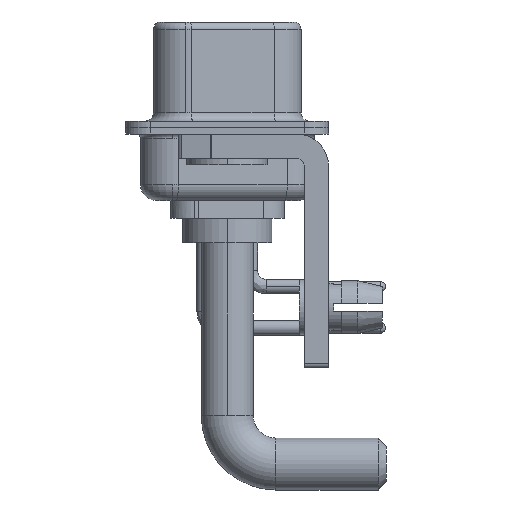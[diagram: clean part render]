
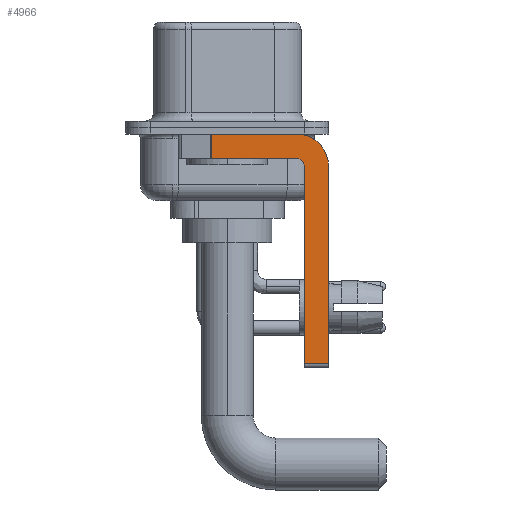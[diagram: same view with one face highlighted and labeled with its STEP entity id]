
A CAD part, left-side view. The second image highlights one B-rep face of the part: STEP entity #4966.
In plain terms, the highlighted planar face has unit normal (-1, 0, 0).
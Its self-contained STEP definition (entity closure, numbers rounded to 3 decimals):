
#356 = EDGE_CURVE ( 'NONE', #11804, #25459, #4008, .T. ) ;
#1149 = CARTESIAN_POINT ( 'NONE',  ( -2.9, 0.978, -1.9 ) ) ;
#2379 = ORIENTED_EDGE ( 'NONE', *, *, #14048, .T. ) ;
#2814 = VECTOR ( 'NONE', #11706, 1000. ) ;
#3312 = DIRECTION ( 'NONE',  ( 0., 0., -1. ) ) ;
#3522 = ORIENTED_EDGE ( 'NONE', *, *, #25595, .F. ) ;
#4008 = LINE ( 'NONE', #19094, #18369 ) ;
#4012 = EDGE_CURVE ( 'NONE', #11804, #10591, #15947, .T. ) ;
#4028 = VECTOR ( 'NONE', #9507, 1000. ) ;
#4048 = DIRECTION ( 'NONE',  ( 0., 0., -1. ) ) ;
#4195 = VERTEX_POINT ( 'NONE', #5942 ) ;
#4743 = ORIENTED_EDGE ( 'NONE', *, *, #9027, .F. ) ;
#4966 = ADVANCED_FACE ( 'NONE', ( #19493 ), #5342, .F. ) ;
#5143 = CARTESIAN_POINT ( 'NONE',  ( -2.9, -4.25, -1.9 ) ) ;
#5342 = PLANE ( 'NONE',  #10728 ) ;
#5614 = CARTESIAN_POINT ( 'NONE',  ( -2.9, -6.25, -2.4 ) ) ;
#5782 = AXIS2_PLACEMENT_3D ( 'NONE', #16795, #25174, #4048 ) ;
#5942 = CARTESIAN_POINT ( 'NONE',  ( -2.9, -4.75, -14.55 ) ) ;
#5973 = DIRECTION ( 'NONE',  ( 0., 1., 0. ) ) ;
#6993 = VECTOR ( 'NONE', #5973, 1000. ) ;
#7260 = CARTESIAN_POINT ( 'NONE',  ( -2.9, -4.25, -2.4 ) ) ;
#7517 = EDGE_LOOP ( 'NONE', ( #22736, #12657, #3522, #9685, #20206, #2379, #23574, #4743 ) ) ;
#8317 = AXIS2_PLACEMENT_3D ( 'NONE', #21967, #15934, #9769 ) ;
#9027 = EDGE_CURVE ( 'NONE', #25459, #19222, #22877, .T. ) ;
#9507 = DIRECTION ( 'NONE',  ( 0., -1., 0. ) ) ;
#9685 = ORIENTED_EDGE ( 'NONE', *, *, #24149, .F. ) ;
#9769 = DIRECTION ( 'NONE',  ( 0., 0., 1. ) ) ;
#9809 = LINE ( 'NONE', #15975, #6993 ) ;
#10589 = EDGE_CURVE ( 'NONE', #4195, #22285, #19416, .T. ) ;
#10591 = VERTEX_POINT ( 'NONE', #10919 ) ;
#10728 = AXIS2_PLACEMENT_3D ( 'NONE', #7260, #17300, #15763 ) ;
#10919 = CARTESIAN_POINT ( 'NONE',  ( -2.9, 0.978, -1.9 ) ) ;
#11208 = CARTESIAN_POINT ( 'NONE',  ( -2.9, -4.25, -0.4 ) ) ;
#11706 = DIRECTION ( 'NONE',  ( 0., 0., -1. ) ) ;
#11804 = VERTEX_POINT ( 'NONE', #25741 ) ;
#11985 = VECTOR ( 'NONE', #12832, 1000. ) ;
#12260 = CIRCLE ( 'NONE', #8317, 0.5 ) ;
#12362 = DIRECTION ( 'NONE',  ( 0., -1., 0. ) ) ;
#12657 = ORIENTED_EDGE ( 'NONE', *, *, #4012, .T. ) ;
#12832 = DIRECTION ( 'NONE',  ( 0., 0., 1. ) ) ;
#14048 = EDGE_CURVE ( 'NONE', #4195, #16558, #25761, .T. ) ;
#14492 = EDGE_CURVE ( 'NONE', #19222, #16558, #17844, .T. ) ;
#15325 = CARTESIAN_POINT ( 'NONE',  ( -2.9, -4.25, -14.55 ) ) ;
#15763 = DIRECTION ( 'NONE',  ( 0., 0., -1. ) ) ;
#15934 = DIRECTION ( 'NONE',  ( -1., 0., 0. ) ) ;
#15947 = LINE ( 'NONE', #1149, #2814 ) ;
#15975 = CARTESIAN_POINT ( 'NONE',  ( -2.9, -4.25, -1.9 ) ) ;
#16197 = VERTEX_POINT ( 'NONE', #5143 ) ;
#16558 = VERTEX_POINT ( 'NONE', #21308 ) ;
#16795 = CARTESIAN_POINT ( 'NONE',  ( -2.9, -4.25, -2.4 ) ) ;
#16901 = CARTESIAN_POINT ( 'NONE',  ( -2.9, -4.75, -2.4 ) ) ;
#17300 = DIRECTION ( 'NONE',  ( 1., 0., 0. ) ) ;
#17363 = CARTESIAN_POINT ( 'NONE',  ( -2.9, -4.75, -14.8 ) ) ;
#17844 = LINE ( 'NONE', #24144, #26385 ) ;
#18369 = VECTOR ( 'NONE', #12362, 1000. ) ;
#19094 = CARTESIAN_POINT ( 'NONE',  ( -2.9, 3., -0.4 ) ) ;
#19222 = VERTEX_POINT ( 'NONE', #5614 ) ;
#19416 = LINE ( 'NONE', #17363, #11985 ) ;
#19493 = FACE_OUTER_BOUND ( 'NONE', #7517, .T. ) ;
#20206 = ORIENTED_EDGE ( 'NONE', *, *, #10589, .F. ) ;
#21308 = CARTESIAN_POINT ( 'NONE',  ( -2.9, -6.25, -14.55 ) ) ;
#21967 = CARTESIAN_POINT ( 'NONE',  ( -2.9, -4.25, -2.4 ) ) ;
#22285 = VERTEX_POINT ( 'NONE', #16901 ) ;
#22736 = ORIENTED_EDGE ( 'NONE', *, *, #356, .F. ) ;
#22877 = CIRCLE ( 'NONE', #5782, 2. ) ;
#23574 = ORIENTED_EDGE ( 'NONE', *, *, #14492, .F. ) ;
#24144 = CARTESIAN_POINT ( 'NONE',  ( -2.9, -6.25, -2.4 ) ) ;
#24149 = EDGE_CURVE ( 'NONE', #22285, #16197, #12260, .T. ) ;
#25174 = DIRECTION ( 'NONE',  ( 1., 0., 0. ) ) ;
#25459 = VERTEX_POINT ( 'NONE', #11208 ) ;
#25595 = EDGE_CURVE ( 'NONE', #16197, #10591, #9809, .T. ) ;
#25741 = CARTESIAN_POINT ( 'NONE',  ( -2.9, 0.978, -0.4 ) ) ;
#25761 = LINE ( 'NONE', #15325, #4028 ) ;
#26385 = VECTOR ( 'NONE', #3312, 1000. ) ;
